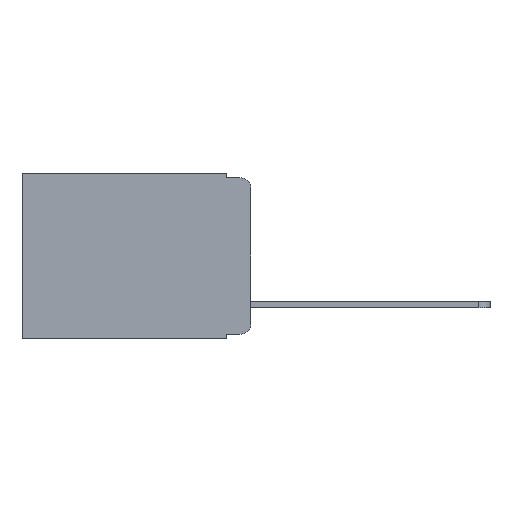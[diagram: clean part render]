
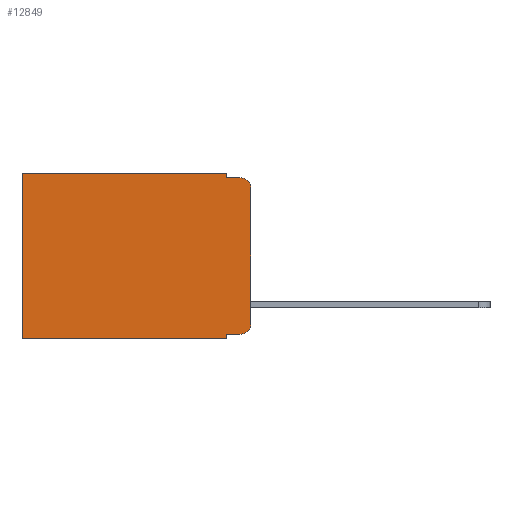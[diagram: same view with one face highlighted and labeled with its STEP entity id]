
A CAD part, left-side view. The second image highlights one B-rep face of the part: STEP entity #12849.
In plain terms, the highlighted planar face has unit normal (-1, 0, 0).
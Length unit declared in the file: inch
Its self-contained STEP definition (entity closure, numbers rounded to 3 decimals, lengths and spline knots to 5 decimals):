
#87 = EDGE_LOOP ( 'NONE', ( #15436, #13559, #4451, #3557, #9933, #3256, #1502, #3498, #8816, #9701 ) ) ;
#150 = AXIS2_PLACEMENT_3D ( 'NONE', #3746, #13528, #2311 ) ;
#347 = VERTEX_POINT ( 'NONE', #4922 ) ;
#496 = VECTOR ( 'NONE', #6916, 39.37008 ) ;
#512 = AXIS2_PLACEMENT_3D ( 'NONE', #17227, #6019, #4553 ) ;
#990 = LINE ( 'NONE', #10602, #4235 ) ;
#1457 = CIRCLE ( 'NONE', #150, 0.02 ) ;
#1502 = ORIENTED_EDGE ( 'NONE', *, *, #13184, .F. ) ;
#1658 = FACE_OUTER_BOUND ( 'NONE', #87, .T. ) ;
#2141 = DIRECTION ( 'NONE',  ( 0., -1., 0. ) ) ;
#2311 = DIRECTION ( 'NONE',  ( 0., 0., -1. ) ) ;
#2484 = CARTESIAN_POINT ( 'NONE',  ( 0.298, 0., -0.03 ) ) ;
#2551 = CARTESIAN_POINT ( 'NONE',  ( 0.298, 0.051, 0. ) ) ;
#2957 = CARTESIAN_POINT ( 'NONE',  ( 0.298, 0.02, -0.313 ) ) ;
#3192 = LINE ( 'NONE', #14905, #5579 ) ;
#3256 = ORIENTED_EDGE ( 'NONE', *, *, #14393, .T. ) ;
#3384 = EDGE_CURVE ( 'NONE', #4462, #14460, #9944, .T. ) ;
#3498 = ORIENTED_EDGE ( 'NONE', *, *, #10571, .F. ) ;
#3557 = ORIENTED_EDGE ( 'NONE', *, *, #3384, .F. ) ;
#3746 = CARTESIAN_POINT ( 'NONE',  ( 0.298, 0.02, -0.03 ) ) ;
#4056 = CARTESIAN_POINT ( 'NONE',  ( 0.298, 0., 0. ) ) ;
#4235 = VECTOR ( 'NONE', #10852, 39.37008 ) ;
#4443 = AXIS2_PLACEMENT_3D ( 'NONE', #2957, #11382, #12718 ) ;
#4451 = ORIENTED_EDGE ( 'NONE', *, *, #10058, .F. ) ;
#4462 = VERTEX_POINT ( 'NONE', #6063 ) ;
#4553 = DIRECTION ( 'NONE',  ( 0., 0., -1. ) ) ;
#4619 = CARTESIAN_POINT ( 'NONE',  ( 0.298, 0.473, 0. ) ) ;
#4661 = PLANE ( 'NONE',  #512 ) ;
#4898 = VECTOR ( 'NONE', #6136, 39.37008 ) ;
#4922 = CARTESIAN_POINT ( 'NONE',  ( 0.298, 0.02, -0.01 ) ) ;
#5003 = VERTEX_POINT ( 'NONE', #7645 ) ;
#5305 = CARTESIAN_POINT ( 'NONE',  ( 0.298, 0., -0.313 ) ) ;
#5547 = VERTEX_POINT ( 'NONE', #7010 ) ;
#5579 = VECTOR ( 'NONE', #15093, 39.37008 ) ;
#5646 = EDGE_CURVE ( 'NONE', #4462, #17533, #17317, .T. ) ;
#6011 = CIRCLE ( 'NONE', #4443, 0.02 ) ;
#6016 = CARTESIAN_POINT ( 'NONE',  ( 0.298, 0.051, 0. ) ) ;
#6019 = DIRECTION ( 'NONE',  ( 1., 0., 0. ) ) ;
#6027 = LINE ( 'NONE', #13302, #13466 ) ;
#6063 = CARTESIAN_POINT ( 'NONE',  ( 0.298, 0.051, 0. ) ) ;
#6136 = DIRECTION ( 'NONE',  ( 0., 0., -1. ) ) ;
#6556 = CARTESIAN_POINT ( 'NONE',  ( 0.298, 0.473, 0. ) ) ;
#6840 = EDGE_CURVE ( 'NONE', #5547, #11527, #9611, .T. ) ;
#6916 = DIRECTION ( 'NONE',  ( 0., 1., 0. ) ) ;
#7010 = CARTESIAN_POINT ( 'NONE',  ( 0.298, 0.051, -0.333 ) ) ;
#7645 = CARTESIAN_POINT ( 'NONE',  ( 0.298, 0.051, -0.343 ) ) ;
#7747 = DIRECTION ( 'NONE',  ( 0., -1., 0. ) ) ;
#7947 = DIRECTION ( 'NONE',  ( 0., 0., -1. ) ) ;
#8063 = VECTOR ( 'NONE', #7747, 39.37008 ) ;
#8816 = ORIENTED_EDGE ( 'NONE', *, *, #6840, .T. ) ;
#9275 = LINE ( 'NONE', #6016, #17618 ) ;
#9445 = VERTEX_POINT ( 'NONE', #5305 ) ;
#9611 = LINE ( 'NONE', #14728, #8063 ) ;
#9701 = ORIENTED_EDGE ( 'NONE', *, *, #11705, .T. ) ;
#9933 = ORIENTED_EDGE ( 'NONE', *, *, #5646, .T. ) ;
#9944 = LINE ( 'NONE', #2551, #12335 ) ;
#10058 = EDGE_CURVE ( 'NONE', #14460, #347, #6027, .T. ) ;
#10248 = DIRECTION ( 'NONE',  ( 0., 0., -1. ) ) ;
#10571 = EDGE_CURVE ( 'NONE', #5547, #5003, #9275, .T. ) ;
#10602 = CARTESIAN_POINT ( 'NONE',  ( 0.298, 0., -0.343 ) ) ;
#10815 = EDGE_CURVE ( 'NONE', #12010, #347, #1457, .T. ) ;
#10852 = DIRECTION ( 'NONE',  ( 0., 1., 0. ) ) ;
#11382 = DIRECTION ( 'NONE',  ( -1., 0., 0. ) ) ;
#11498 = EDGE_CURVE ( 'NONE', #12010, #9445, #3192, .T. ) ;
#11527 = VERTEX_POINT ( 'NONE', #15421 ) ;
#11705 = EDGE_CURVE ( 'NONE', #11527, #9445, #6011, .T. ) ;
#11924 = LINE ( 'NONE', #4619, #4898 ) ;
#12010 = VERTEX_POINT ( 'NONE', #2484 ) ;
#12335 = VECTOR ( 'NONE', #7947, 39.37008 ) ;
#12718 = DIRECTION ( 'NONE',  ( 0., 0., -1. ) ) ;
#12849 = ADVANCED_FACE ( 'NONE', ( #1658 ), #4661, .F. ) ;
#13184 = EDGE_CURVE ( 'NONE', #5003, #16068, #990, .T. ) ;
#13302 = CARTESIAN_POINT ( 'NONE',  ( 0.298, 0.051, -0.01 ) ) ;
#13466 = VECTOR ( 'NONE', #2141, 39.37008 ) ;
#13528 = DIRECTION ( 'NONE',  ( -1., 0., 0. ) ) ;
#13559 = ORIENTED_EDGE ( 'NONE', *, *, #10815, .T. ) ;
#14393 = EDGE_CURVE ( 'NONE', #17533, #16068, #11924, .T. ) ;
#14460 = VERTEX_POINT ( 'NONE', #17719 ) ;
#14728 = CARTESIAN_POINT ( 'NONE',  ( 0.298, 0.051, -0.333 ) ) ;
#14905 = CARTESIAN_POINT ( 'NONE',  ( 0.298, 0., 0. ) ) ;
#15093 = DIRECTION ( 'NONE',  ( 0., 0., -1. ) ) ;
#15265 = CARTESIAN_POINT ( 'NONE',  ( 0.298, 0.473, -0.343 ) ) ;
#15421 = CARTESIAN_POINT ( 'NONE',  ( 0.298, 0.02, -0.333 ) ) ;
#15436 = ORIENTED_EDGE ( 'NONE', *, *, #11498, .F. ) ;
#16068 = VERTEX_POINT ( 'NONE', #15265 ) ;
#17227 = CARTESIAN_POINT ( 'NONE',  ( 0.298, 0., 0. ) ) ;
#17317 = LINE ( 'NONE', #4056, #496 ) ;
#17533 = VERTEX_POINT ( 'NONE', #6556 ) ;
#17618 = VECTOR ( 'NONE', #10248, 39.37008 ) ;
#17719 = CARTESIAN_POINT ( 'NONE',  ( 0.298, 0.051, -0.01 ) ) ;
